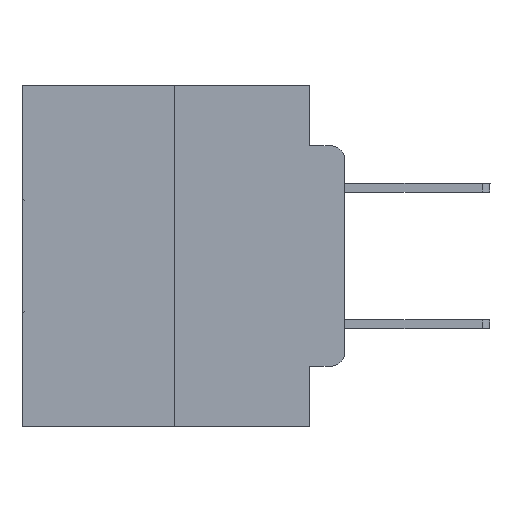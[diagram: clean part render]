
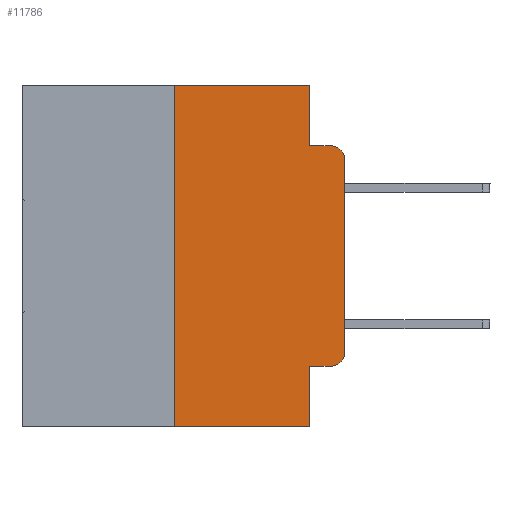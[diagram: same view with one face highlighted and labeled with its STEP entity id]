
A CAD part, left-side view. The second image highlights one B-rep face of the part: STEP entity #11786.
In plain terms, the highlighted planar face has unit normal (-1, 0, 0).
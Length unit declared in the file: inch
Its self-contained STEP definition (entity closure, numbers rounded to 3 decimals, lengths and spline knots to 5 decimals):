
#78 = VERTEX_POINT ( 'NONE', #1081 ) ;
#696 = VECTOR ( 'NONE', #9993, 39.37008 ) ;
#893 = ORIENTED_EDGE ( 'NONE', *, *, #25661, .F. ) ;
#1017 = CARTESIAN_POINT ( 'NONE',  ( 0., 0.25, -0.5 ) ) ;
#1061 = CIRCLE ( 'NONE', #6279, 0.02 ) ;
#1081 = CARTESIAN_POINT ( 'NONE',  ( 0., 0.051, -0.5 ) ) ;
#1318 = EDGE_LOOP ( 'NONE', ( #28785, #13298, #22920, #25460, #22815, #25040, #16436, #893, #4815, #13653 ) ) ;
#1444 = DIRECTION ( 'NONE',  ( 0., 0., -1. ) ) ;
#2431 = CARTESIAN_POINT ( 'NONE',  ( 0., 0.473, 0. ) ) ;
#2989 = VECTOR ( 'NONE', #22465, 39.37008 ) ;
#3608 = EDGE_CURVE ( 'NONE', #20249, #25668, #26754, .T. ) ;
#4305 = DIRECTION ( 'NONE',  ( 0., 0., 1. ) ) ;
#4375 = DIRECTION ( 'NONE',  ( 1., 0., 0. ) ) ;
#4815 = ORIENTED_EDGE ( 'NONE', *, *, #13177, .T. ) ;
#4963 = CARTESIAN_POINT ( 'NONE',  ( 0., 0.051, -0.0885 ) ) ;
#5609 = EDGE_CURVE ( 'NONE', #9330, #10968, #6678, .T. ) ;
#5661 = CARTESIAN_POINT ( 'NONE',  ( 0., 0., -0.3915 ) ) ;
#6199 = CARTESIAN_POINT ( 'NONE',  ( 0., 0.02, -0.1085 ) ) ;
#6279 = AXIS2_PLACEMENT_3D ( 'NONE', #22475, #26904, #11345 ) ;
#6583 = CARTESIAN_POINT ( 'NONE',  ( 0., 0.051, -0.4115 ) ) ;
#6678 = LINE ( 'NONE', #24615, #25975 ) ;
#7169 = VERTEX_POINT ( 'NONE', #18550 ) ;
#8030 = AXIS2_PLACEMENT_3D ( 'NONE', #6199, #28740, #1444 ) ;
#8504 = CIRCLE ( 'NONE', #8030, 0.02 ) ;
#8999 = CARTESIAN_POINT ( 'NONE',  ( 0., 0.02, -0.0885 ) ) ;
#9114 = DIRECTION ( 'NONE',  ( 0., 0., -1. ) ) ;
#9330 = VERTEX_POINT ( 'NONE', #5661 ) ;
#9739 = VERTEX_POINT ( 'NONE', #1017 ) ;
#9993 = DIRECTION ( 'NONE',  ( 0., 0., 1. ) ) ;
#10734 = VERTEX_POINT ( 'NONE', #4963 ) ;
#10911 = CARTESIAN_POINT ( 'NONE',  ( 0., 0.02, -0.4115 ) ) ;
#10968 = VERTEX_POINT ( 'NONE', #15192 ) ;
#11345 = DIRECTION ( 'NONE',  ( 0., 0., -1. ) ) ;
#11786 = ADVANCED_FACE ( 'NONE', ( #26910 ), #15813, .F. ) ;
#12510 = LINE ( 'NONE', #18882, #19654 ) ;
#12979 = DIRECTION ( 'NONE',  ( 0., -1., 0. ) ) ;
#13177 = EDGE_CURVE ( 'NONE', #7169, #26694, #26892, .T. ) ;
#13298 = ORIENTED_EDGE ( 'NONE', *, *, #27898, .T. ) ;
#13653 = ORIENTED_EDGE ( 'NONE', *, *, #21630, .T. ) ;
#14144 = CARTESIAN_POINT ( 'NONE',  ( 0., 0.051, 0. ) ) ;
#14512 = CARTESIAN_POINT ( 'NONE',  ( 0., 0.051, -0.0885 ) ) ;
#15192 = CARTESIAN_POINT ( 'NONE',  ( 0., 0., -0.1085 ) ) ;
#15478 = CARTESIAN_POINT ( 'NONE',  ( 0., 0.473, 0. ) ) ;
#15813 = PLANE ( 'NONE',  #23860 ) ;
#16436 = ORIENTED_EDGE ( 'NONE', *, *, #21531, .T. ) ;
#16874 = LINE ( 'NONE', #14512, #19558 ) ;
#18550 = CARTESIAN_POINT ( 'NONE',  ( 0., 0.051, -0.4115 ) ) ;
#18882 = CARTESIAN_POINT ( 'NONE',  ( 0., 0.051, 0. ) ) ;
#18966 = VECTOR ( 'NONE', #9114, 39.37008 ) ;
#19558 = VECTOR ( 'NONE', #23682, 39.37008 ) ;
#19654 = VECTOR ( 'NONE', #28368, 39.37008 ) ;
#20249 = VERTEX_POINT ( 'NONE', #28067 ) ;
#20971 = VECTOR ( 'NONE', #26775, 39.37008 ) ;
#21531 = EDGE_CURVE ( 'NONE', #9739, #78, #21602, .T. ) ;
#21602 = LINE ( 'NONE', #22041, #20971 ) ;
#21630 = EDGE_CURVE ( 'NONE', #26694, #9330, #1061, .T. ) ;
#21651 = VECTOR ( 'NONE', #12979, 39.37008 ) ;
#22041 = CARTESIAN_POINT ( 'NONE',  ( 0., 0.473, -0.5 ) ) ;
#22465 = DIRECTION ( 'NONE',  ( 0., -1., 0. ) ) ;
#22475 = CARTESIAN_POINT ( 'NONE',  ( 0., 0.02, -0.3915 ) ) ;
#22815 = ORIENTED_EDGE ( 'NONE', *, *, #3608, .F. ) ;
#22884 = CARTESIAN_POINT ( 'NONE',  ( 0., 0.051, 0. ) ) ;
#22920 = ORIENTED_EDGE ( 'NONE', *, *, #23746, .F. ) ;
#23682 = DIRECTION ( 'NONE',  ( 0., -1., 0. ) ) ;
#23746 = EDGE_CURVE ( 'NONE', #10734, #28107, #16874, .T. ) ;
#23860 = AXIS2_PLACEMENT_3D ( 'NONE', #2431, #4375, #24684 ) ;
#24615 = CARTESIAN_POINT ( 'NONE',  ( 0., 0., 0. ) ) ;
#24684 = DIRECTION ( 'NONE',  ( 0., 0., -1. ) ) ;
#25040 = ORIENTED_EDGE ( 'NONE', *, *, #25581, .F. ) ;
#25395 = LINE ( 'NONE', #22884, #18966 ) ;
#25460 = ORIENTED_EDGE ( 'NONE', *, *, #26795, .F. ) ;
#25541 = CARTESIAN_POINT ( 'NONE',  ( 0., 0.25, 0. ) ) ;
#25581 = EDGE_CURVE ( 'NONE', #9739, #20249, #25981, .T. ) ;
#25661 = EDGE_CURVE ( 'NONE', #7169, #78, #12510, .T. ) ;
#25668 = VERTEX_POINT ( 'NONE', #14144 ) ;
#25975 = VECTOR ( 'NONE', #4305, 39.37008 ) ;
#25981 = LINE ( 'NONE', #25541, #696 ) ;
#26694 = VERTEX_POINT ( 'NONE', #10911 ) ;
#26754 = LINE ( 'NONE', #15478, #21651 ) ;
#26775 = DIRECTION ( 'NONE',  ( 0., -1., 0. ) ) ;
#26795 = EDGE_CURVE ( 'NONE', #25668, #10734, #25395, .T. ) ;
#26892 = LINE ( 'NONE', #6583, #2989 ) ;
#26904 = DIRECTION ( 'NONE',  ( -1., 0., 0. ) ) ;
#26910 = FACE_OUTER_BOUND ( 'NONE', #1318, .T. ) ;
#27898 = EDGE_CURVE ( 'NONE', #10968, #28107, #8504, .T. ) ;
#28067 = CARTESIAN_POINT ( 'NONE',  ( 0., 0.25, 0. ) ) ;
#28107 = VERTEX_POINT ( 'NONE', #8999 ) ;
#28368 = DIRECTION ( 'NONE',  ( 0., 0., -1. ) ) ;
#28740 = DIRECTION ( 'NONE',  ( -1., 0., 0. ) ) ;
#28785 = ORIENTED_EDGE ( 'NONE', *, *, #5609, .T. ) ;
